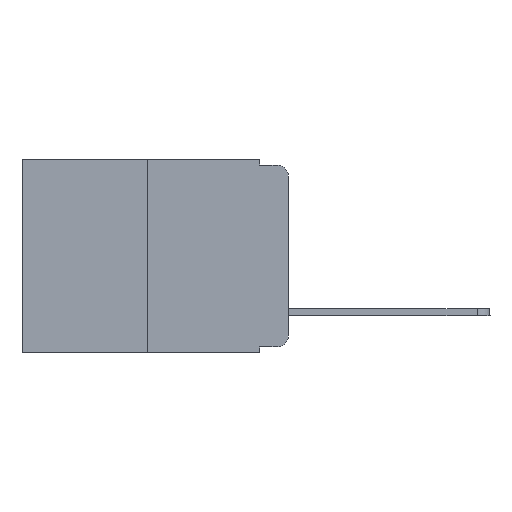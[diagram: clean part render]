
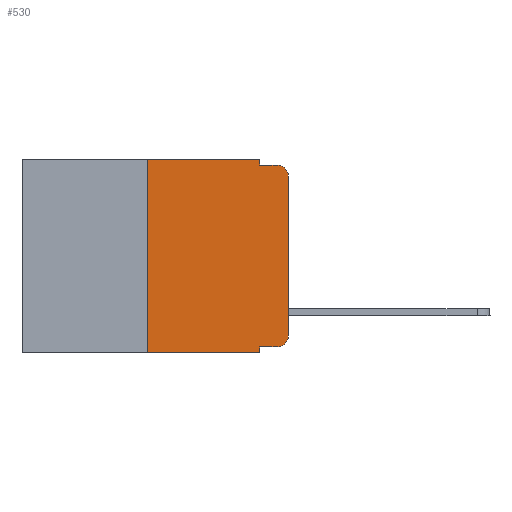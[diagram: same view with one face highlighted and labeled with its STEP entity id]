
A CAD part, left-side view. The second image highlights one B-rep face of the part: STEP entity #530.
In plain terms, the highlighted planar face has unit normal (-1, 0, 0).
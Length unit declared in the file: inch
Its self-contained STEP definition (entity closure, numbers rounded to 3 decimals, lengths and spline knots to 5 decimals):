
#331 = DIRECTION ( 'NONE',  ( 0., -1., 0. ) ) ;
#525 = DIRECTION ( 'NONE',  ( -1., 0., 0. ) ) ;
#530 = ADVANCED_FACE ( 'NONE', ( #9087 ), #12312, .F. ) ;
#586 = AXIS2_PLACEMENT_3D ( 'NONE', #7251, #525, #11754 ) ;
#617 = DIRECTION ( 'NONE',  ( 0., -1., 0. ) ) ;
#686 = DIRECTION ( 'NONE',  ( 0., -1., 0. ) ) ;
#804 = LINE ( 'NONE', #11351, #11622 ) ;
#849 = DIRECTION ( 'NONE',  ( 0., 0., -1. ) ) ;
#1435 = CARTESIAN_POINT ( 'NONE',  ( 0., 0.473, -0.343 ) ) ;
#1444 = ORIENTED_EDGE ( 'NONE', *, *, #11951, .T. ) ;
#1843 = ORIENTED_EDGE ( 'NONE', *, *, #3111, .F. ) ;
#1862 = VERTEX_POINT ( 'NONE', #4429 ) ;
#2352 = VERTEX_POINT ( 'NONE', #7673 ) ;
#2487 = VERTEX_POINT ( 'NONE', #5487 ) ;
#2597 = ORIENTED_EDGE ( 'NONE', *, *, #9992, .T. ) ;
#2669 = AXIS2_PLACEMENT_3D ( 'NONE', #8786, #9901, #13228 ) ;
#2787 = CARTESIAN_POINT ( 'NONE',  ( 0., 0., 0. ) ) ;
#2942 = CARTESIAN_POINT ( 'NONE',  ( 0., 0.051, -0.01 ) ) ;
#2967 = CARTESIAN_POINT ( 'NONE',  ( 0., 0.02, -0.03 ) ) ;
#3022 = ORIENTED_EDGE ( 'NONE', *, *, #7963, .T. ) ;
#3035 = VERTEX_POINT ( 'NONE', #6064 ) ;
#3111 = EDGE_CURVE ( 'NONE', #5517, #2487, #9488, .T. ) ;
#3196 = LINE ( 'NONE', #1435, #7676 ) ;
#3328 = CIRCLE ( 'NONE', #586, 0.02 ) ;
#4425 = CARTESIAN_POINT ( 'NONE',  ( 0., 0.25, -0.343 ) ) ;
#4429 = CARTESIAN_POINT ( 'NONE',  ( 0., 0., -0.313 ) ) ;
#4701 = DIRECTION ( 'NONE',  ( 0., -1., 0. ) ) ;
#4717 = EDGE_CURVE ( 'NONE', #1862, #10095, #8812, .T. ) ;
#4998 = AXIS2_PLACEMENT_3D ( 'NONE', #2967, #13063, #10724 ) ;
#5230 = VERTEX_POINT ( 'NONE', #4425 ) ;
#5389 = EDGE_CURVE ( 'NONE', #5983, #3035, #804, .T. ) ;
#5468 = VECTOR ( 'NONE', #12346, 39.37008 ) ;
#5487 = CARTESIAN_POINT ( 'NONE',  ( 0., 0.02, -0.01 ) ) ;
#5517 = VERTEX_POINT ( 'NONE', #2942 ) ;
#5559 = LINE ( 'NONE', #11662, #14262 ) ;
#5865 = CARTESIAN_POINT ( 'NONE',  ( 0., 0.25, 0. ) ) ;
#5924 = ORIENTED_EDGE ( 'NONE', *, *, #5389, .F. ) ;
#5983 = VERTEX_POINT ( 'NONE', #5865 ) ;
#6032 = CIRCLE ( 'NONE', #4998, 0.02 ) ;
#6064 = CARTESIAN_POINT ( 'NONE',  ( 0., 0.051, 0. ) ) ;
#6087 = EDGE_CURVE ( 'NONE', #3035, #5517, #7380, .T. ) ;
#6160 = EDGE_CURVE ( 'NONE', #5230, #5983, #6487, .T. ) ;
#6252 = ORIENTED_EDGE ( 'NONE', *, *, #7388, .F. ) ;
#6487 = LINE ( 'NONE', #7948, #5468 ) ;
#7130 = CARTESIAN_POINT ( 'NONE',  ( 0., 0.051, -0.333 ) ) ;
#7251 = CARTESIAN_POINT ( 'NONE',  ( 0., 0.02, -0.313 ) ) ;
#7362 = CARTESIAN_POINT ( 'NONE',  ( 0., 0.051, -0.01 ) ) ;
#7380 = LINE ( 'NONE', #8672, #9491 ) ;
#7388 = EDGE_CURVE ( 'NONE', #12658, #2352, #9809, .T. ) ;
#7670 = ORIENTED_EDGE ( 'NONE', *, *, #11978, .T. ) ;
#7673 = CARTESIAN_POINT ( 'NONE',  ( 0., 0.051, -0.343 ) ) ;
#7676 = VECTOR ( 'NONE', #331, 39.37008 ) ;
#7948 = CARTESIAN_POINT ( 'NONE',  ( 0., 0.25, 0. ) ) ;
#7963 = EDGE_CURVE ( 'NONE', #10095, #2487, #6032, .T. ) ;
#8042 = CARTESIAN_POINT ( 'NONE',  ( 0., 0.02, -0.333 ) ) ;
#8340 = ORIENTED_EDGE ( 'NONE', *, *, #6160, .F. ) ;
#8672 = CARTESIAN_POINT ( 'NONE',  ( 0., 0.051, 0. ) ) ;
#8786 = CARTESIAN_POINT ( 'NONE',  ( 0., 0.473, 0. ) ) ;
#8812 = LINE ( 'NONE', #2787, #10743 ) ;
#9087 = FACE_OUTER_BOUND ( 'NONE', #11341, .T. ) ;
#9488 = LINE ( 'NONE', #7362, #13855 ) ;
#9491 = VECTOR ( 'NONE', #849, 39.37008 ) ;
#9809 = LINE ( 'NONE', #11242, #10182 ) ;
#9901 = DIRECTION ( 'NONE',  ( 1., 0., 0. ) ) ;
#9992 = EDGE_CURVE ( 'NONE', #5230, #2352, #3196, .T. ) ;
#10095 = VERTEX_POINT ( 'NONE', #12627 ) ;
#10182 = VECTOR ( 'NONE', #12354, 39.37008 ) ;
#10407 = DIRECTION ( 'NONE',  ( 0., 0., 1. ) ) ;
#10724 = DIRECTION ( 'NONE',  ( 0., 0., -1. ) ) ;
#10743 = VECTOR ( 'NONE', #10407, 39.37008 ) ;
#11242 = CARTESIAN_POINT ( 'NONE',  ( 0., 0.051, 0. ) ) ;
#11341 = EDGE_LOOP ( 'NONE', ( #11915, #3022, #1843, #11833, #5924, #8340, #2597, #6252, #7670, #1444 ) ) ;
#11351 = CARTESIAN_POINT ( 'NONE',  ( 0., 0.473, 0. ) ) ;
#11622 = VECTOR ( 'NONE', #4701, 39.37008 ) ;
#11662 = CARTESIAN_POINT ( 'NONE',  ( 0., 0.051, -0.333 ) ) ;
#11754 = DIRECTION ( 'NONE',  ( 0., 0., -1. ) ) ;
#11833 = ORIENTED_EDGE ( 'NONE', *, *, #6087, .F. ) ;
#11915 = ORIENTED_EDGE ( 'NONE', *, *, #4717, .T. ) ;
#11951 = EDGE_CURVE ( 'NONE', #13261, #1862, #3328, .T. ) ;
#11978 = EDGE_CURVE ( 'NONE', #12658, #13261, #5559, .T. ) ;
#12312 = PLANE ( 'NONE',  #2669 ) ;
#12346 = DIRECTION ( 'NONE',  ( 0., 0., 1. ) ) ;
#12354 = DIRECTION ( 'NONE',  ( 0., 0., -1. ) ) ;
#12627 = CARTESIAN_POINT ( 'NONE',  ( 0., 0., -0.03 ) ) ;
#12658 = VERTEX_POINT ( 'NONE', #7130 ) ;
#13063 = DIRECTION ( 'NONE',  ( -1., 0., 0. ) ) ;
#13228 = DIRECTION ( 'NONE',  ( 0., 0., -1. ) ) ;
#13261 = VERTEX_POINT ( 'NONE', #8042 ) ;
#13855 = VECTOR ( 'NONE', #686, 39.37008 ) ;
#14262 = VECTOR ( 'NONE', #617, 39.37008 ) ;
